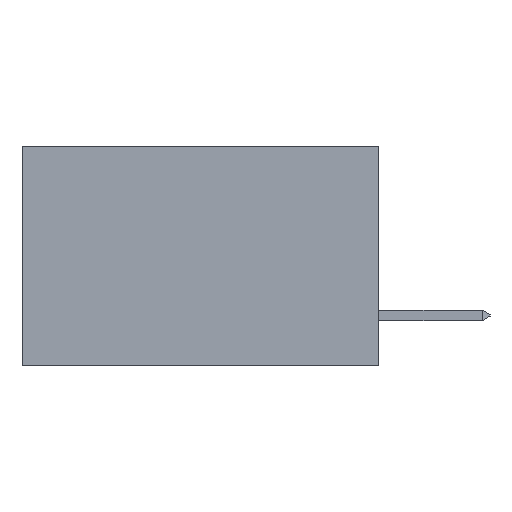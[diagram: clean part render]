
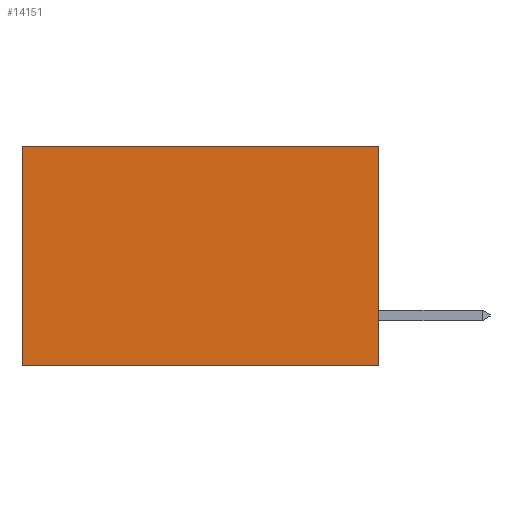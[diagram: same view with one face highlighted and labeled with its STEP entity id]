
A CAD part, left-side view. The second image highlights one B-rep face of the part: STEP entity #14151.
In plain terms, the highlighted planar face has unit normal (-1, 0, 0).
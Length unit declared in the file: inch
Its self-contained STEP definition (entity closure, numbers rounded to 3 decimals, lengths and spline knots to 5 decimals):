
#540 = CARTESIAN_POINT ( 'NONE',  ( 0.2615, 0.6, 0. ) ) ;
#679 = EDGE_CURVE ( 'NONE', #19219, #20044, #15587, .T. ) ;
#1347 = ORIENTED_EDGE ( 'NONE', *, *, #4682, .T. ) ;
#1784 = VECTOR ( 'NONE', #16483, 39.37008 ) ;
#2236 = VERTEX_POINT ( 'NONE', #4247 ) ;
#3076 = LINE ( 'NONE', #8986, #11735 ) ;
#3152 = ORIENTED_EDGE ( 'NONE', *, *, #679, .F. ) ;
#4247 = CARTESIAN_POINT ( 'NONE',  ( 0.2615, 0., 0. ) ) ;
#4265 = VECTOR ( 'NONE', #17837, 39.37008 ) ;
#4372 = ORIENTED_EDGE ( 'NONE', *, *, #12366, .F. ) ;
#4682 = EDGE_CURVE ( 'NONE', #2236, #12577, #8919, .T. ) ;
#5918 = EDGE_LOOP ( 'NONE', ( #20266, #3152, #4372, #1347 ) ) ;
#6067 = CARTESIAN_POINT ( 'NONE',  ( 0.2615, 0., -0.37 ) ) ;
#6252 = FACE_OUTER_BOUND ( 'NONE', #5918, .T. ) ;
#6342 = VECTOR ( 'NONE', #14108, 39.37008 ) ;
#6893 = LINE ( 'NONE', #14629, #6342 ) ;
#8552 = CARTESIAN_POINT ( 'NONE',  ( 0.2615, 0., -0.37 ) ) ;
#8716 = DIRECTION ( 'NONE',  ( 0., 0., -1. ) ) ;
#8919 = LINE ( 'NONE', #17982, #4265 ) ;
#8986 = CARTESIAN_POINT ( 'NONE',  ( 0.2615, 0.6, -0.37 ) ) ;
#11735 = VECTOR ( 'NONE', #8716, 39.37008 ) ;
#12366 = EDGE_CURVE ( 'NONE', #2236, #19219, #6893, .T. ) ;
#12577 = VERTEX_POINT ( 'NONE', #540 ) ;
#13885 = AXIS2_PLACEMENT_3D ( 'NONE', #16858, #16645, #16518 ) ;
#13897 = EDGE_CURVE ( 'NONE', #12577, #20044, #3076, .T. ) ;
#14108 = DIRECTION ( 'NONE',  ( 0., 0., -1. ) ) ;
#14151 = ADVANCED_FACE ( 'NONE', ( #6252 ), #16876, .F. ) ;
#14629 = CARTESIAN_POINT ( 'NONE',  ( 0.2615, 0., -0.37 ) ) ;
#15587 = LINE ( 'NONE', #8552, #1784 ) ;
#16483 = DIRECTION ( 'NONE',  ( 0., 1., 0. ) ) ;
#16518 = DIRECTION ( 'NONE',  ( 0., 0., -1. ) ) ;
#16645 = DIRECTION ( 'NONE',  ( 1., 0., 0. ) ) ;
#16858 = CARTESIAN_POINT ( 'NONE',  ( 0.2615, 0., -0.37 ) ) ;
#16876 = PLANE ( 'NONE',  #13885 ) ;
#16939 = CARTESIAN_POINT ( 'NONE',  ( 0.2615, 0.6, -0.37 ) ) ;
#17837 = DIRECTION ( 'NONE',  ( 0., 1., 0. ) ) ;
#17982 = CARTESIAN_POINT ( 'NONE',  ( 0.2615, 0., 0. ) ) ;
#19219 = VERTEX_POINT ( 'NONE', #6067 ) ;
#20044 = VERTEX_POINT ( 'NONE', #16939 ) ;
#20266 = ORIENTED_EDGE ( 'NONE', *, *, #13897, .T. ) ;
